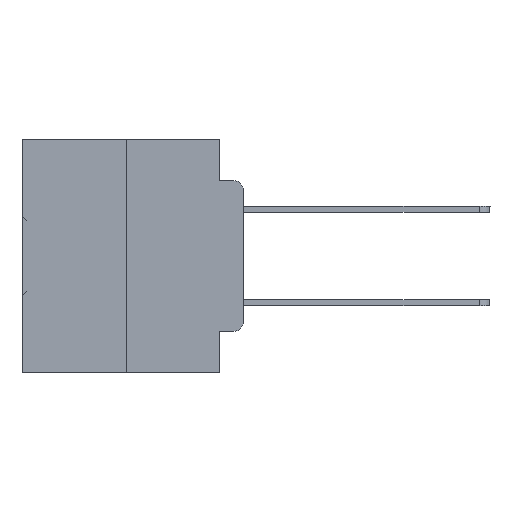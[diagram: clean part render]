
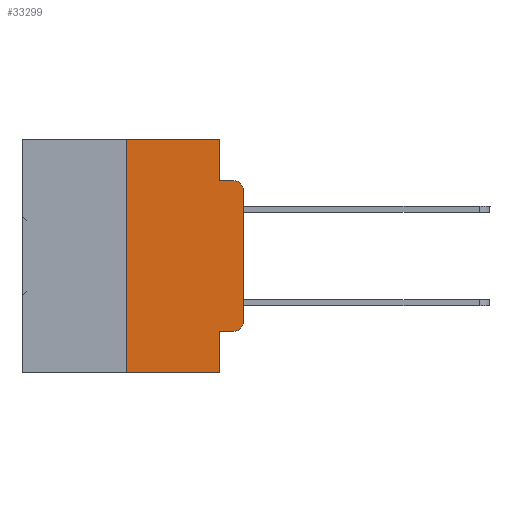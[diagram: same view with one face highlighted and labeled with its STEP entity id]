
A CAD part, left-side view. The second image highlights one B-rep face of the part: STEP entity #33299.
In plain terms, the highlighted planar face has unit normal (-1, 0, 0).
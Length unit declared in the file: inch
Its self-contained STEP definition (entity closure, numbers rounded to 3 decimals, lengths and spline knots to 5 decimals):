
#3746 = CARTESIAN_POINT ( 'NONE',  ( 0., 0.051, 0. ) ) ;
#3972 = ORIENTED_EDGE ( 'NONE', *, *, #30598, .T. ) ;
#4202 = CARTESIAN_POINT ( 'NONE',  ( 0., 0., 0. ) ) ;
#5017 = VECTOR ( 'NONE', #29057, 39.37008 ) ;
#5038 = CARTESIAN_POINT ( 'NONE',  ( 0., 0.051, 0. ) ) ;
#5461 = EDGE_CURVE ( 'NONE', #25388, #25366, #28732, .T. ) ;
#5476 = EDGE_CURVE ( 'NONE', #37655, #9557, #14656, .T. ) ;
#5923 = VERTEX_POINT ( 'NONE', #16567 ) ;
#5956 = CARTESIAN_POINT ( 'NONE',  ( 0., 0.473, 0. ) ) ;
#6023 = CARTESIAN_POINT ( 'NONE',  ( 0., 0.25, -0.5 ) ) ;
#6127 = AXIS2_PLACEMENT_3D ( 'NONE', #26752, #20097, #38060 ) ;
#6348 = ORIENTED_EDGE ( 'NONE', *, *, #17507, .F. ) ;
#6915 = VERTEX_POINT ( 'NONE', #11601 ) ;
#7811 = LINE ( 'NONE', #19692, #22326 ) ;
#9138 = CARTESIAN_POINT ( 'NONE',  ( 0., 0.051, -0.5 ) ) ;
#9299 = CARTESIAN_POINT ( 'NONE',  ( 0., 0.051, -0.4115 ) ) ;
#9557 = VERTEX_POINT ( 'NONE', #3746 ) ;
#10054 = DIRECTION ( 'NONE',  ( 0., 0., 1. ) ) ;
#10883 = CIRCLE ( 'NONE', #22055, 0.02 ) ;
#11363 = EDGE_CURVE ( 'NONE', #17630, #28749, #18699, .T. ) ;
#11473 = EDGE_LOOP ( 'NONE', ( #31409, #3972, #17064, #18769, #15267, #26825, #35875, #6348, #14729, #38143 ) ) ;
#11601 = CARTESIAN_POINT ( 'NONE',  ( 0., 0., -0.3915 ) ) ;
#12209 = CARTESIAN_POINT ( 'NONE',  ( 0., 0.051, 0. ) ) ;
#12488 = DIRECTION ( 'NONE',  ( 0., -1., 0. ) ) ;
#13370 = DIRECTION ( 'NONE',  ( 0., 0., -1. ) ) ;
#13923 = CARTESIAN_POINT ( 'NONE',  ( 0., 0.02, -0.0885 ) ) ;
#14656 = LINE ( 'NONE', #23818, #15311 ) ;
#14729 = ORIENTED_EDGE ( 'NONE', *, *, #27758, .T. ) ;
#15267 = ORIENTED_EDGE ( 'NONE', *, *, #5476, .F. ) ;
#15311 = VECTOR ( 'NONE', #35917, 39.37008 ) ;
#15845 = EDGE_CURVE ( 'NONE', #5923, #6915, #34813, .T. ) ;
#16497 = VERTEX_POINT ( 'NONE', #9299 ) ;
#16567 = CARTESIAN_POINT ( 'NONE',  ( 0., 0.02, -0.4115 ) ) ;
#16775 = DIRECTION ( 'NONE',  ( 0., 0., 1. ) ) ;
#16822 = VECTOR ( 'NONE', #24104, 39.37008 ) ;
#17064 = ORIENTED_EDGE ( 'NONE', *, *, #11363, .F. ) ;
#17087 = DIRECTION ( 'NONE',  ( 0., 0., -1. ) ) ;
#17130 = LINE ( 'NONE', #5038, #5017 ) ;
#17507 = EDGE_CURVE ( 'NONE', #16497, #25366, #33474, .T. ) ;
#17630 = VERTEX_POINT ( 'NONE', #24880 ) ;
#18499 = DIRECTION ( 'NONE',  ( 0., -1., 0. ) ) ;
#18699 = LINE ( 'NONE', #30622, #19570 ) ;
#18769 = ORIENTED_EDGE ( 'NONE', *, *, #35025, .F. ) ;
#19570 = VECTOR ( 'NONE', #18499, 39.37008 ) ;
#19692 = CARTESIAN_POINT ( 'NONE',  ( 0., 0.25, 0. ) ) ;
#19707 = CARTESIAN_POINT ( 'NONE',  ( 0., 0., -0.1085 ) ) ;
#20097 = DIRECTION ( 'NONE',  ( -1., 0., 0. ) ) ;
#20672 = EDGE_CURVE ( 'NONE', #6915, #32900, #30355, .T. ) ;
#20767 = PLANE ( 'NONE',  #37844 ) ;
#22055 = AXIS2_PLACEMENT_3D ( 'NONE', #37384, #28417, #13370 ) ;
#22326 = VECTOR ( 'NONE', #16775, 39.37008 ) ;
#22944 = FACE_OUTER_BOUND ( 'NONE', #11473, .T. ) ;
#23818 = CARTESIAN_POINT ( 'NONE',  ( 0., 0.473, 0. ) ) ;
#24104 = DIRECTION ( 'NONE',  ( 0., 0., -1. ) ) ;
#24579 = LINE ( 'NONE', #36483, #35729 ) ;
#24880 = CARTESIAN_POINT ( 'NONE',  ( 0., 0.051, -0.0885 ) ) ;
#25366 = VERTEX_POINT ( 'NONE', #9138 ) ;
#25388 = VERTEX_POINT ( 'NONE', #6023 ) ;
#26002 = CARTESIAN_POINT ( 'NONE',  ( 0., 0.473, -0.5 ) ) ;
#26752 = CARTESIAN_POINT ( 'NONE',  ( 0., 0.02, -0.3915 ) ) ;
#26825 = ORIENTED_EDGE ( 'NONE', *, *, #36153, .F. ) ;
#27758 = EDGE_CURVE ( 'NONE', #16497, #5923, #24579, .T. ) ;
#28417 = DIRECTION ( 'NONE',  ( -1., 0., 0. ) ) ;
#28732 = LINE ( 'NONE', #26002, #35880 ) ;
#28749 = VERTEX_POINT ( 'NONE', #13923 ) ;
#29057 = DIRECTION ( 'NONE',  ( 0., 0., -1. ) ) ;
#30355 = LINE ( 'NONE', #4202, #31240 ) ;
#30598 = EDGE_CURVE ( 'NONE', #32900, #28749, #10883, .T. ) ;
#30622 = CARTESIAN_POINT ( 'NONE',  ( 0., 0.051, -0.0885 ) ) ;
#31240 = VECTOR ( 'NONE', #10054, 39.37008 ) ;
#31409 = ORIENTED_EDGE ( 'NONE', *, *, #20672, .T. ) ;
#32685 = DIRECTION ( 'NONE',  ( 1., 0., 0. ) ) ;
#32900 = VERTEX_POINT ( 'NONE', #19707 ) ;
#33299 = ADVANCED_FACE ( 'NONE', ( #22944 ), #20767, .F. ) ;
#33474 = LINE ( 'NONE', #12209, #16822 ) ;
#34813 = CIRCLE ( 'NONE', #6127, 0.02 ) ;
#35025 = EDGE_CURVE ( 'NONE', #9557, #17630, #17130, .T. ) ;
#35729 = VECTOR ( 'NONE', #12488, 39.37008 ) ;
#35875 = ORIENTED_EDGE ( 'NONE', *, *, #5461, .T. ) ;
#35880 = VECTOR ( 'NONE', #37890, 39.37008 ) ;
#35917 = DIRECTION ( 'NONE',  ( 0., -1., 0. ) ) ;
#36153 = EDGE_CURVE ( 'NONE', #25388, #37655, #7811, .T. ) ;
#36483 = CARTESIAN_POINT ( 'NONE',  ( 0., 0.051, -0.4115 ) ) ;
#37384 = CARTESIAN_POINT ( 'NONE',  ( 0., 0.02, -0.1085 ) ) ;
#37655 = VERTEX_POINT ( 'NONE', #38424 ) ;
#37844 = AXIS2_PLACEMENT_3D ( 'NONE', #5956, #32685, #17087 ) ;
#37890 = DIRECTION ( 'NONE',  ( 0., -1., 0. ) ) ;
#38060 = DIRECTION ( 'NONE',  ( 0., 0., -1. ) ) ;
#38143 = ORIENTED_EDGE ( 'NONE', *, *, #15845, .T. ) ;
#38424 = CARTESIAN_POINT ( 'NONE',  ( 0., 0.25, 0. ) ) ;
